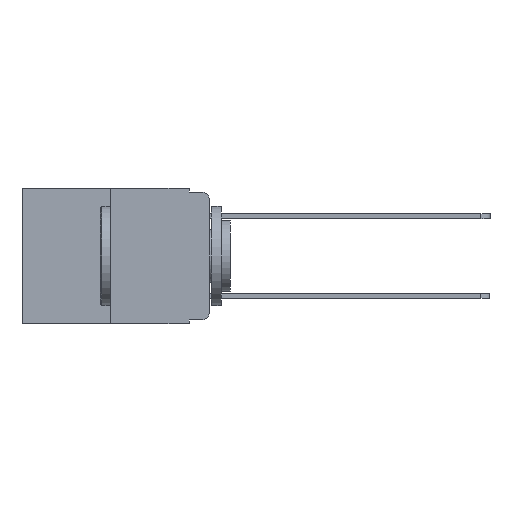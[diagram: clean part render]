
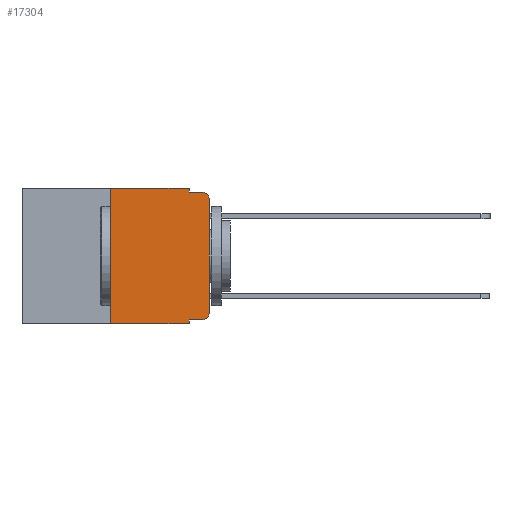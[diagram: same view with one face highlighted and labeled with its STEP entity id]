
A CAD part, left-side view. The second image highlights one B-rep face of the part: STEP entity #17304.
In plain terms, the highlighted planar face has unit normal (-1, 0, 0).
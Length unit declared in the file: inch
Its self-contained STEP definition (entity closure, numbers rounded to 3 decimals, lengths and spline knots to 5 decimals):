
#442 = CIRCLE ( 'NONE', #20042, 0.02 ) ;
#502 = CARTESIAN_POINT ( 'NONE',  ( 0., 0.473, -0.343 ) ) ;
#985 = CARTESIAN_POINT ( 'NONE',  ( 0., 0.051, 0. ) ) ;
#2061 = VECTOR ( 'NONE', #16900, 39.37008 ) ;
#2241 = VERTEX_POINT ( 'NONE', #12488 ) ;
#2274 = VECTOR ( 'NONE', #20422, 39.37008 ) ;
#2346 = LINE ( 'NONE', #13878, #10758 ) ;
#2541 = LINE ( 'NONE', #8340, #14724 ) ;
#2662 = CARTESIAN_POINT ( 'NONE',  ( 0., 0.051, 0. ) ) ;
#2832 = CARTESIAN_POINT ( 'NONE',  ( 0., 0., -0.03 ) ) ;
#3164 = DIRECTION ( 'NONE',  ( -1., 0., 0. ) ) ;
#3476 = ORIENTED_EDGE ( 'NONE', *, *, #19603, .F. ) ;
#3730 = ORIENTED_EDGE ( 'NONE', *, *, #14939, .F. ) ;
#4061 = VERTEX_POINT ( 'NONE', #7691 ) ;
#4113 = CARTESIAN_POINT ( 'NONE',  ( 0., 0.473, 0. ) ) ;
#4210 = CARTESIAN_POINT ( 'NONE',  ( 0., 0.25, 0. ) ) ;
#4915 = ORIENTED_EDGE ( 'NONE', *, *, #9564, .T. ) ;
#5097 = ORIENTED_EDGE ( 'NONE', *, *, #20126, .T. ) ;
#5510 = CARTESIAN_POINT ( 'NONE',  ( 0., 0.25, 0. ) ) ;
#5659 = DIRECTION ( 'NONE',  ( 0., -1., 0. ) ) ;
#5757 = CIRCLE ( 'NONE', #19254, 0.02 ) ;
#5843 = DIRECTION ( 'NONE',  ( 0., 0., -1. ) ) ;
#5930 = DIRECTION ( 'NONE',  ( 0., 0., 1. ) ) ;
#6573 = VERTEX_POINT ( 'NONE', #985 ) ;
#6731 = CARTESIAN_POINT ( 'NONE',  ( 0., 0.051, 0. ) ) ;
#7691 = CARTESIAN_POINT ( 'NONE',  ( 0., 0.02, -0.333 ) ) ;
#7717 = DIRECTION ( 'NONE',  ( -1., 0., 0. ) ) ;
#7782 = LINE ( 'NONE', #2662, #2274 ) ;
#7934 = ORIENTED_EDGE ( 'NONE', *, *, #11759, .T. ) ;
#8211 = ORIENTED_EDGE ( 'NONE', *, *, #12873, .F. ) ;
#8212 = LINE ( 'NONE', #4210, #16304 ) ;
#8340 = CARTESIAN_POINT ( 'NONE',  ( 0., 0., 0. ) ) ;
#8660 = DIRECTION ( 'NONE',  ( 0., -1., 0. ) ) ;
#9028 = ORIENTED_EDGE ( 'NONE', *, *, #12044, .T. ) ;
#9191 = CARTESIAN_POINT ( 'NONE',  ( 0., 0.051, -0.01 ) ) ;
#9564 = EDGE_CURVE ( 'NONE', #4061, #18874, #442, .T. ) ;
#9618 = ORIENTED_EDGE ( 'NONE', *, *, #20160, .T. ) ;
#9722 = VECTOR ( 'NONE', #5659, 39.37008 ) ;
#9864 = CARTESIAN_POINT ( 'NONE',  ( 0., 0.02, -0.01 ) ) ;
#10045 = LINE ( 'NONE', #6731, #17947 ) ;
#10078 = DIRECTION ( 'NONE',  ( 0., 0., 1. ) ) ;
#10234 = LINE ( 'NONE', #502, #9722 ) ;
#10639 = VERTEX_POINT ( 'NONE', #5510 ) ;
#10758 = VECTOR ( 'NONE', #15387, 39.37008 ) ;
#10819 = PLANE ( 'NONE',  #19604 ) ;
#11759 = EDGE_CURVE ( 'NONE', #19000, #4061, #15228, .T. ) ;
#12044 = EDGE_CURVE ( 'NONE', #21051, #2241, #10234, .T. ) ;
#12278 = VERTEX_POINT ( 'NONE', #2832 ) ;
#12488 = CARTESIAN_POINT ( 'NONE',  ( 0., 0.051, -0.343 ) ) ;
#12873 = EDGE_CURVE ( 'NONE', #19000, #2241, #7782, .T. ) ;
#13223 = CARTESIAN_POINT ( 'NONE',  ( 0., 0.02, -0.03 ) ) ;
#13364 = LINE ( 'NONE', #19754, #16955 ) ;
#13878 = CARTESIAN_POINT ( 'NONE',  ( 0., 0.051, -0.01 ) ) ;
#14501 = VERTEX_POINT ( 'NONE', #9191 ) ;
#14724 = VECTOR ( 'NONE', #10078, 39.37008 ) ;
#14762 = DIRECTION ( 'NONE',  ( 0., 0., -1. ) ) ;
#14939 = EDGE_CURVE ( 'NONE', #21051, #10639, #8212, .T. ) ;
#15228 = LINE ( 'NONE', #15333, #2061 ) ;
#15333 = CARTESIAN_POINT ( 'NONE',  ( 0., 0.051, -0.333 ) ) ;
#15387 = DIRECTION ( 'NONE',  ( 0., -1., 0. ) ) ;
#15620 = DIRECTION ( 'NONE',  ( 1., 0., 0. ) ) ;
#16304 = VECTOR ( 'NONE', #5930, 39.37008 ) ;
#16720 = FACE_OUTER_BOUND ( 'NONE', #19447, .T. ) ;
#16739 = CARTESIAN_POINT ( 'NONE',  ( 0., 0.051, -0.333 ) ) ;
#16900 = DIRECTION ( 'NONE',  ( 0., -1., 0. ) ) ;
#16955 = VECTOR ( 'NONE', #8660, 39.37008 ) ;
#17026 = EDGE_CURVE ( 'NONE', #6573, #14501, #10045, .T. ) ;
#17304 = ADVANCED_FACE ( 'NONE', ( #16720 ), #10819, .F. ) ;
#17394 = CARTESIAN_POINT ( 'NONE',  ( 0., 0.02, -0.313 ) ) ;
#17686 = CARTESIAN_POINT ( 'NONE',  ( 0., 0.25, -0.343 ) ) ;
#17700 = CARTESIAN_POINT ( 'NONE',  ( 0., 0., -0.313 ) ) ;
#17947 = VECTOR ( 'NONE', #19607, 39.37008 ) ;
#18874 = VERTEX_POINT ( 'NONE', #17700 ) ;
#18925 = DIRECTION ( 'NONE',  ( 0., 0., -1. ) ) ;
#19000 = VERTEX_POINT ( 'NONE', #16739 ) ;
#19081 = EDGE_CURVE ( 'NONE', #14501, #19416, #2346, .T. ) ;
#19254 = AXIS2_PLACEMENT_3D ( 'NONE', #13223, #3164, #14762 ) ;
#19416 = VERTEX_POINT ( 'NONE', #9864 ) ;
#19439 = ORIENTED_EDGE ( 'NONE', *, *, #17026, .F. ) ;
#19447 = EDGE_LOOP ( 'NONE', ( #9618, #5097, #20806, #19439, #3476, #3730, #9028, #8211, #7934, #4915 ) ) ;
#19603 = EDGE_CURVE ( 'NONE', #10639, #6573, #13364, .T. ) ;
#19604 = AXIS2_PLACEMENT_3D ( 'NONE', #4113, #15620, #5843 ) ;
#19607 = DIRECTION ( 'NONE',  ( 0., 0., -1. ) ) ;
#19754 = CARTESIAN_POINT ( 'NONE',  ( 0., 0.473, 0. ) ) ;
#20042 = AXIS2_PLACEMENT_3D ( 'NONE', #17394, #7717, #18925 ) ;
#20126 = EDGE_CURVE ( 'NONE', #12278, #19416, #5757, .T. ) ;
#20160 = EDGE_CURVE ( 'NONE', #18874, #12278, #2541, .T. ) ;
#20422 = DIRECTION ( 'NONE',  ( 0., 0., -1. ) ) ;
#20806 = ORIENTED_EDGE ( 'NONE', *, *, #19081, .F. ) ;
#21051 = VERTEX_POINT ( 'NONE', #17686 ) ;
